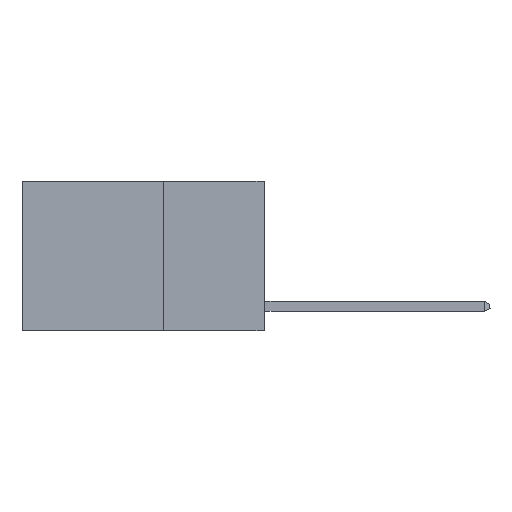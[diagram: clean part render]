
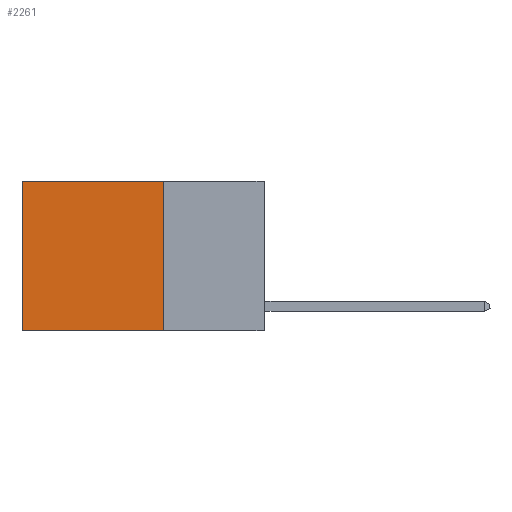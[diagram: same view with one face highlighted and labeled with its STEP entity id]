
A CAD part, left-side view. The second image highlights one B-rep face of the part: STEP entity #2261.
In plain terms, the highlighted planar face has unit normal (-1, 0, 0).
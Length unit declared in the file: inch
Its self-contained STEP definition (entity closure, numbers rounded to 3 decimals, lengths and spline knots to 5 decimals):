
#486 = DIRECTION ( 'NONE',  ( 1., 0., 0. ) ) ;
#1864 = CARTESIAN_POINT ( 'NONE',  ( 0.2625, 0.25, 0. ) ) ;
#2261 = ADVANCED_FACE ( 'NONE', ( #7559 ), #8801, .F. ) ;
#2301 = EDGE_LOOP ( 'NONE', ( #3262, #12378, #11555, #2456 ) ) ;
#2456 = ORIENTED_EDGE ( 'NONE', *, *, #6513, .T. ) ;
#2458 = LINE ( 'NONE', #12032, #13076 ) ;
#2652 = VECTOR ( 'NONE', #7830, 39.37008 ) ;
#3262 = ORIENTED_EDGE ( 'NONE', *, *, #16446, .T. ) ;
#4177 = CARTESIAN_POINT ( 'NONE',  ( 0.2625, 0.6, 0. ) ) ;
#4257 = VECTOR ( 'NONE', #5672, 39.37008 ) ;
#4776 = VERTEX_POINT ( 'NONE', #1864 ) ;
#4972 = EDGE_CURVE ( 'NONE', #4776, #5939, #2458, .T. ) ;
#5110 = CARTESIAN_POINT ( 'NONE',  ( 0.2625, 0.25, 0. ) ) ;
#5638 = EDGE_CURVE ( 'NONE', #5939, #6792, #6318, .T. ) ;
#5672 = DIRECTION ( 'NONE',  ( 0., 0., -1. ) ) ;
#5939 = VERTEX_POINT ( 'NONE', #9456 ) ;
#6284 = LINE ( 'NONE', #5110, #17686 ) ;
#6318 = LINE ( 'NONE', #17464, #2652 ) ;
#6513 = EDGE_CURVE ( 'NONE', #4776, #16381, #6284, .T. ) ;
#6792 = VERTEX_POINT ( 'NONE', #8831 ) ;
#7559 = FACE_OUTER_BOUND ( 'NONE', #2301, .T. ) ;
#7830 = DIRECTION ( 'NONE',  ( 0., 1., 0. ) ) ;
#7911 = DIRECTION ( 'NONE',  ( 0., 0., -1. ) ) ;
#8801 = PLANE ( 'NONE',  #16418 ) ;
#8831 = CARTESIAN_POINT ( 'NONE',  ( 0.2625, 0.6, -0.37 ) ) ;
#9456 = CARTESIAN_POINT ( 'NONE',  ( 0.2625, 0.25, -0.37 ) ) ;
#10203 = DIRECTION ( 'NONE',  ( 0., 0., -1. ) ) ;
#11555 = ORIENTED_EDGE ( 'NONE', *, *, #4972, .F. ) ;
#11644 = LINE ( 'NONE', #13981, #4257 ) ;
#12032 = CARTESIAN_POINT ( 'NONE',  ( 0.2625, 0.25, 0. ) ) ;
#12378 = ORIENTED_EDGE ( 'NONE', *, *, #5638, .F. ) ;
#13076 = VECTOR ( 'NONE', #7911, 39.37008 ) ;
#13981 = CARTESIAN_POINT ( 'NONE',  ( 0.2625, 0.6, 0. ) ) ;
#15633 = CARTESIAN_POINT ( 'NONE',  ( 0.2625, 0.25, 0. ) ) ;
#16127 = DIRECTION ( 'NONE',  ( 0., 1., 0. ) ) ;
#16381 = VERTEX_POINT ( 'NONE', #4177 ) ;
#16418 = AXIS2_PLACEMENT_3D ( 'NONE', #15633, #486, #10203 ) ;
#16446 = EDGE_CURVE ( 'NONE', #16381, #6792, #11644, .T. ) ;
#17464 = CARTESIAN_POINT ( 'NONE',  ( 0.2625, 0.25, -0.37 ) ) ;
#17686 = VECTOR ( 'NONE', #16127, 39.37008 ) ;
